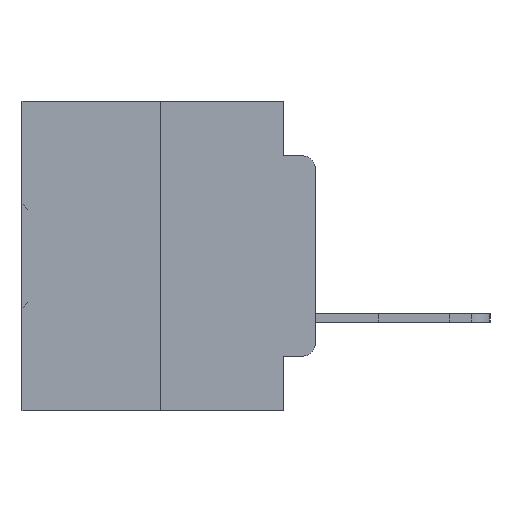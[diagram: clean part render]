
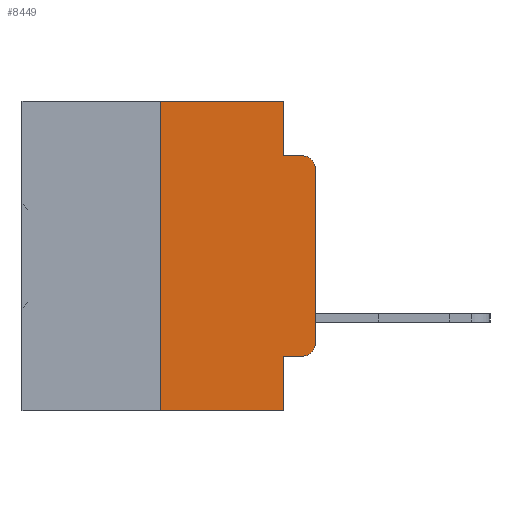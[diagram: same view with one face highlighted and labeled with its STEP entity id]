
A CAD part, left-side view. The second image highlights one B-rep face of the part: STEP entity #8449.
In plain terms, the highlighted planar face has unit normal (-1, 0, 0).
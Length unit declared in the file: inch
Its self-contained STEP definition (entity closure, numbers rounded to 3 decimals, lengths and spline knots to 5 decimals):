
#1170 = EDGE_CURVE ( 'NONE', #33629, #15942, #26729, .T. ) ;
#1257 = DIRECTION ( 'NONE',  ( 0., 0., 1. ) ) ;
#1543 = DIRECTION ( 'NONE',  ( 0., -1., 0. ) ) ;
#1777 = DIRECTION ( 'NONE',  ( 0., -1., 0. ) ) ;
#2240 = CIRCLE ( 'NONE', #17216, 0.02 ) ;
#2243 = VECTOR ( 'NONE', #17333, 39.37008 ) ;
#2427 = FACE_OUTER_BOUND ( 'NONE', #11515, .T. ) ;
#2998 = VECTOR ( 'NONE', #20200, 39.37008 ) ;
#3006 = CARTESIAN_POINT ( 'NONE',  ( 0., 0.02, -0.4115 ) ) ;
#4251 = ORIENTED_EDGE ( 'NONE', *, *, #14568, .F. ) ;
#5438 = CARTESIAN_POINT ( 'NONE',  ( 0., 0.02, -0.3915 ) ) ;
#5634 = VERTEX_POINT ( 'NONE', #23562 ) ;
#5661 = CARTESIAN_POINT ( 'NONE',  ( 0., 0., -0.3915 ) ) ;
#6062 = EDGE_CURVE ( 'NONE', #18564, #8925, #17552, .T. ) ;
#6226 = CARTESIAN_POINT ( 'NONE',  ( 0., 0.02, -0.0885 ) ) ;
#6909 = ORIENTED_EDGE ( 'NONE', *, *, #1170, .T. ) ;
#7624 = VERTEX_POINT ( 'NONE', #5661 ) ;
#8268 = DIRECTION ( 'NONE',  ( 0., 0., -1. ) ) ;
#8415 = VECTOR ( 'NONE', #1257, 39.37008 ) ;
#8449 = ADVANCED_FACE ( 'NONE', ( #2427 ), #25165, .F. ) ;
#8506 = CARTESIAN_POINT ( 'NONE',  ( 0., 0.473, -0.5 ) ) ;
#8608 = DIRECTION ( 'NONE',  ( 1., 0., 0. ) ) ;
#8925 = VERTEX_POINT ( 'NONE', #27830 ) ;
#8944 = CARTESIAN_POINT ( 'NONE',  ( 0., 0.051, -0.0885 ) ) ;
#9190 = AXIS2_PLACEMENT_3D ( 'NONE', #17202, #8608, #27757 ) ;
#9220 = CARTESIAN_POINT ( 'NONE',  ( 0., 0.051, -0.4115 ) ) ;
#9648 = ORIENTED_EDGE ( 'NONE', *, *, #28806, .T. ) ;
#9696 = VECTOR ( 'NONE', #27677, 39.37008 ) ;
#9925 = EDGE_CURVE ( 'NONE', #13238, #33581, #14306, .T. ) ;
#10131 = CARTESIAN_POINT ( 'NONE',  ( 0., 0.473, 0. ) ) ;
#10435 = VECTOR ( 'NONE', #21568, 39.37008 ) ;
#10542 = ORIENTED_EDGE ( 'NONE', *, *, #15062, .T. ) ;
#10727 = CARTESIAN_POINT ( 'NONE',  ( 0., 0.051, -0.4115 ) ) ;
#10883 = EDGE_CURVE ( 'NONE', #34786, #18564, #12850, .T. ) ;
#11007 = ORIENTED_EDGE ( 'NONE', *, *, #6062, .F. ) ;
#11515 = EDGE_LOOP ( 'NONE', ( #10542, #22244, #14207, #11007, #15997, #4251, #21023, #13778, #6909, #9648 ) ) ;
#11562 = CARTESIAN_POINT ( 'NONE',  ( 0., 0.051, 0. ) ) ;
#12689 = LINE ( 'NONE', #8944, #19246 ) ;
#12850 = LINE ( 'NONE', #10131, #32572 ) ;
#13238 = VERTEX_POINT ( 'NONE', #27614 ) ;
#13778 = ORIENTED_EDGE ( 'NONE', *, *, #27926, .F. ) ;
#14207 = ORIENTED_EDGE ( 'NONE', *, *, #32419, .F. ) ;
#14306 = CIRCLE ( 'NONE', #32465, 0.02 ) ;
#14568 = EDGE_CURVE ( 'NONE', #5634, #34786, #30185, .T. ) ;
#14707 = CARTESIAN_POINT ( 'NONE',  ( 0., 0.051, 0. ) ) ;
#15062 = EDGE_CURVE ( 'NONE', #7624, #13238, #24409, .T. ) ;
#15942 = VERTEX_POINT ( 'NONE', #3006 ) ;
#15997 = ORIENTED_EDGE ( 'NONE', *, *, #10883, .F. ) ;
#15998 = CARTESIAN_POINT ( 'NONE',  ( 0., 0.02, -0.1085 ) ) ;
#16226 = CARTESIAN_POINT ( 'NONE',  ( 0., 0.051, 0. ) ) ;
#17202 = CARTESIAN_POINT ( 'NONE',  ( 0., 0.473, 0. ) ) ;
#17216 = AXIS2_PLACEMENT_3D ( 'NONE', #5438, #24870, #8268 ) ;
#17333 = DIRECTION ( 'NONE',  ( 0., 0., -1. ) ) ;
#17552 = LINE ( 'NONE', #11562, #2243 ) ;
#17719 = EDGE_CURVE ( 'NONE', #5634, #19737, #30522, .T. ) ;
#18564 = VERTEX_POINT ( 'NONE', #14707 ) ;
#18733 = DIRECTION ( 'NONE',  ( 0., 0., -1. ) ) ;
#19246 = VECTOR ( 'NONE', #30736, 39.37008 ) ;
#19737 = VERTEX_POINT ( 'NONE', #24953 ) ;
#19752 = VECTOR ( 'NONE', #1777, 39.37008 ) ;
#20200 = DIRECTION ( 'NONE',  ( 0., 0., 1. ) ) ;
#21023 = ORIENTED_EDGE ( 'NONE', *, *, #17719, .T. ) ;
#21568 = DIRECTION ( 'NONE',  ( 0., 0., -1. ) ) ;
#22244 = ORIENTED_EDGE ( 'NONE', *, *, #9925, .T. ) ;
#23562 = CARTESIAN_POINT ( 'NONE',  ( 0., 0.25, -0.5 ) ) ;
#24409 = LINE ( 'NONE', #28530, #2998 ) ;
#24870 = DIRECTION ( 'NONE',  ( -1., 0., 0. ) ) ;
#24953 = CARTESIAN_POINT ( 'NONE',  ( 0., 0.051, -0.5 ) ) ;
#25045 = LINE ( 'NONE', #16226, #10435 ) ;
#25165 = PLANE ( 'NONE',  #9190 ) ;
#26729 = LINE ( 'NONE', #10727, #19752 ) ;
#27614 = CARTESIAN_POINT ( 'NONE',  ( 0., 0., -0.1085 ) ) ;
#27677 = DIRECTION ( 'NONE',  ( 0., -1., 0. ) ) ;
#27757 = DIRECTION ( 'NONE',  ( 0., 0., -1. ) ) ;
#27830 = CARTESIAN_POINT ( 'NONE',  ( 0., 0.051, -0.0885 ) ) ;
#27926 = EDGE_CURVE ( 'NONE', #33629, #19737, #25045, .T. ) ;
#28530 = CARTESIAN_POINT ( 'NONE',  ( 0., 0., 0. ) ) ;
#28806 = EDGE_CURVE ( 'NONE', #15942, #7624, #2240, .T. ) ;
#30185 = LINE ( 'NONE', #34245, #8415 ) ;
#30522 = LINE ( 'NONE', #8506, #9696 ) ;
#30675 = CARTESIAN_POINT ( 'NONE',  ( 0., 0.25, 0. ) ) ;
#30736 = DIRECTION ( 'NONE',  ( 0., -1., 0. ) ) ;
#32419 = EDGE_CURVE ( 'NONE', #8925, #33581, #12689, .T. ) ;
#32465 = AXIS2_PLACEMENT_3D ( 'NONE', #15998, #34538, #18733 ) ;
#32572 = VECTOR ( 'NONE', #1543, 39.37008 ) ;
#33581 = VERTEX_POINT ( 'NONE', #6226 ) ;
#33629 = VERTEX_POINT ( 'NONE', #9220 ) ;
#34245 = CARTESIAN_POINT ( 'NONE',  ( 0., 0.25, 0. ) ) ;
#34538 = DIRECTION ( 'NONE',  ( -1., 0., 0. ) ) ;
#34786 = VERTEX_POINT ( 'NONE', #30675 ) ;
